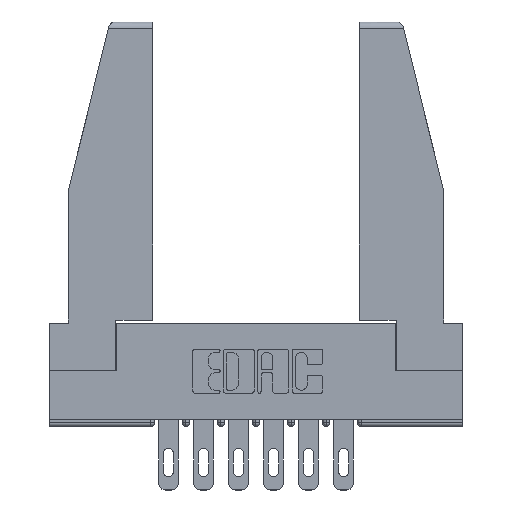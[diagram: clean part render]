
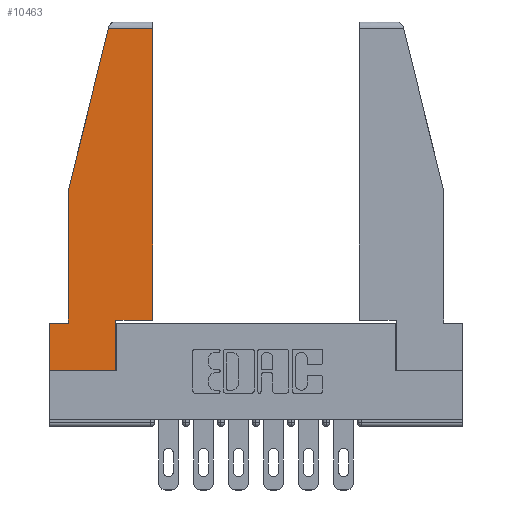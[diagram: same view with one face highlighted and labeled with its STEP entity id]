
A CAD part, top view. The second image highlights one B-rep face of the part: STEP entity #10463.
In plain terms, the highlighted planar face has unit normal (0, 0, 1).
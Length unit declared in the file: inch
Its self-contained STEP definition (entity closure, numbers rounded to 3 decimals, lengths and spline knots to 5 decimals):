
#146 = VERTEX_POINT ( 'NONE', #12851 ) ;
#574 = ORIENTED_EDGE ( 'NONE', *, *, #5669, .T. ) ;
#767 = DIRECTION ( 'NONE',  ( 1., 0., 0. ) ) ;
#911 = VERTEX_POINT ( 'NONE', #9817 ) ;
#975 = EDGE_LOOP ( 'NONE', ( #574, #4840, #1830, #4346, #2373, #11514, #5509, #6616, #11898 ) ) ;
#1115 = DIRECTION ( 'NONE',  ( 0., 0., 1. ) ) ;
#1830 = ORIENTED_EDGE ( 'NONE', *, *, #10739, .T. ) ;
#2018 = LINE ( 'NONE', #5982, #3346 ) ;
#2109 = CARTESIAN_POINT ( 'NONE',  ( 0., 0.21, 0. ) ) ;
#2373 = ORIENTED_EDGE ( 'NONE', *, *, #6642, .T. ) ;
#2510 = CARTESIAN_POINT ( 'NONE',  ( 0.297, 0.223, 0. ) ) ;
#2668 = CARTESIAN_POINT ( 'NONE',  ( 0.297, 0., 0. ) ) ;
#2847 = LINE ( 'NONE', #8634, #6261 ) ;
#2888 = DIRECTION ( 'NONE',  ( -1., 0., 0. ) ) ;
#3025 = CARTESIAN_POINT ( 'NONE',  ( 0.461, 0.223, 0. ) ) ;
#3156 = VERTEX_POINT ( 'NONE', #2668 ) ;
#3254 = DIRECTION ( 'NONE',  ( 0., 1., 0. ) ) ;
#3298 = CARTESIAN_POINT ( 'NONE',  ( 0.2636, 1.52, 0. ) ) ;
#3346 = VECTOR ( 'NONE', #5923, 39.37008 ) ;
#3618 = DIRECTION ( 'NONE',  ( 1., 0., 0. ) ) ;
#3627 = VERTEX_POINT ( 'NONE', #4947 ) ;
#3676 = DIRECTION ( 'NONE',  ( 0., -1., 0. ) ) ;
#3731 = CARTESIAN_POINT ( 'NONE',  ( 0., 0.21, 0. ) ) ;
#3956 = AXIS2_PLACEMENT_3D ( 'NONE', #9051, #1115, #8014 ) ;
#3998 = VECTOR ( 'NONE', #3254, 39.37008 ) ;
#4346 = ORIENTED_EDGE ( 'NONE', *, *, #10928, .T. ) ;
#4360 = CARTESIAN_POINT ( 'NONE',  ( 0.086, 0.8, 0. ) ) ;
#4773 = EDGE_CURVE ( 'NONE', #3156, #911, #6033, .T. ) ;
#4840 = ORIENTED_EDGE ( 'NONE', *, *, #7980, .T. ) ;
#4947 = CARTESIAN_POINT ( 'NONE',  ( 0., 0., 0. ) ) ;
#5002 = VECTOR ( 'NONE', #3618, 39.37008 ) ;
#5118 = EDGE_CURVE ( 'NONE', #3627, #3156, #2847, .T. ) ;
#5456 = VECTOR ( 'NONE', #10964, 39.37008 ) ;
#5509 = ORIENTED_EDGE ( 'NONE', *, *, #5118, .T. ) ;
#5585 = VERTEX_POINT ( 'NONE', #9003 ) ;
#5669 = EDGE_CURVE ( 'NONE', #5585, #146, #10831, .T. ) ;
#5763 = CARTESIAN_POINT ( 'NONE',  ( 0., 0.21, 0. ) ) ;
#5923 = DIRECTION ( 'NONE',  ( 0., -1., 0. ) ) ;
#5962 = VERTEX_POINT ( 'NONE', #4360 ) ;
#5982 = CARTESIAN_POINT ( 'NONE',  ( 0.086, 0.8, 0. ) ) ;
#6033 = LINE ( 'NONE', #6100, #3998 ) ;
#6100 = CARTESIAN_POINT ( 'NONE',  ( 0.297, 0., 0. ) ) ;
#6261 = VECTOR ( 'NONE', #767, 39.37008 ) ;
#6616 = ORIENTED_EDGE ( 'NONE', *, *, #4773, .T. ) ;
#6642 = EDGE_CURVE ( 'NONE', #11808, #9201, #7021, .T. ) ;
#6656 = LINE ( 'NONE', #5763, #11449 ) ;
#6758 = CARTESIAN_POINT ( 'NONE',  ( 0.271, 1.55, 0. ) ) ;
#7021 = LINE ( 'NONE', #3731, #10097 ) ;
#7646 = VERTEX_POINT ( 'NONE', #3298 ) ;
#7695 = DIRECTION ( 'NONE',  ( -1., 0., 0. ) ) ;
#7839 = CARTESIAN_POINT ( 'NONE',  ( 0.086, 0.21, 0. ) ) ;
#7980 = EDGE_CURVE ( 'NONE', #146, #7646, #10906, .T. ) ;
#8014 = DIRECTION ( 'NONE',  ( 1., 0., 0. ) ) ;
#8217 = VECTOR ( 'NONE', #2888, 39.37008 ) ;
#8634 = CARTESIAN_POINT ( 'NONE',  ( 0., 0., 0. ) ) ;
#8696 = LINE ( 'NONE', #2510, #5002 ) ;
#9003 = CARTESIAN_POINT ( 'NONE',  ( 0.461, 0.223, 0. ) ) ;
#9051 = CARTESIAN_POINT ( 'NONE',  ( 0., 0., 0. ) ) ;
#9201 = VERTEX_POINT ( 'NONE', #2109 ) ;
#9817 = CARTESIAN_POINT ( 'NONE',  ( 0.297, 0.223, 0. ) ) ;
#9835 = LINE ( 'NONE', #6758, #12500 ) ;
#10097 = VECTOR ( 'NONE', #7695, 39.37008 ) ;
#10193 = EDGE_CURVE ( 'NONE', #911, #5585, #8696, .T. ) ;
#10463 = ADVANCED_FACE ( 'NONE', ( #11941 ), #11070, .T. ) ;
#10739 = EDGE_CURVE ( 'NONE', #7646, #5962, #9835, .T. ) ;
#10831 = LINE ( 'NONE', #3025, #5456 ) ;
#10906 = LINE ( 'NONE', #11826, #8217 ) ;
#10928 = EDGE_CURVE ( 'NONE', #5962, #11808, #2018, .T. ) ;
#10964 = DIRECTION ( 'NONE',  ( 0., 1., 0. ) ) ;
#11070 = PLANE ( 'NONE',  #3956 ) ;
#11449 = VECTOR ( 'NONE', #3676, 39.37008 ) ;
#11514 = ORIENTED_EDGE ( 'NONE', *, *, #12849, .T. ) ;
#11729 = DIRECTION ( 'NONE',  ( -0.239, -0.971, 0. ) ) ;
#11808 = VERTEX_POINT ( 'NONE', #7839 ) ;
#11826 = CARTESIAN_POINT ( 'NONE',  ( 0., 1.52, 0. ) ) ;
#11898 = ORIENTED_EDGE ( 'NONE', *, *, #10193, .T. ) ;
#11941 = FACE_OUTER_BOUND ( 'NONE', #975, .T. ) ;
#12500 = VECTOR ( 'NONE', #11729, 39.37008 ) ;
#12849 = EDGE_CURVE ( 'NONE', #9201, #3627, #6656, .T. ) ;
#12851 = CARTESIAN_POINT ( 'NONE',  ( 0.461, 1.52, 0. ) ) ;
